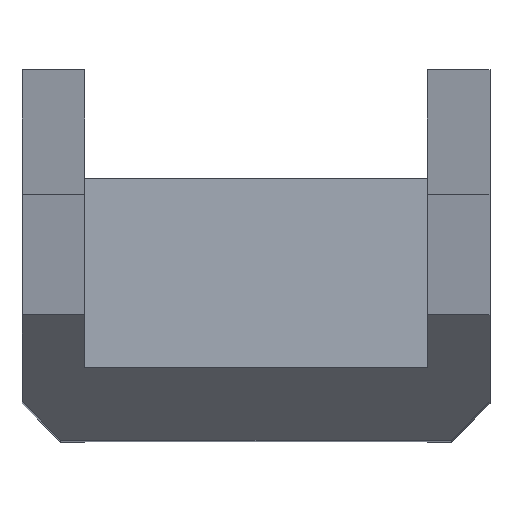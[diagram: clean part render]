
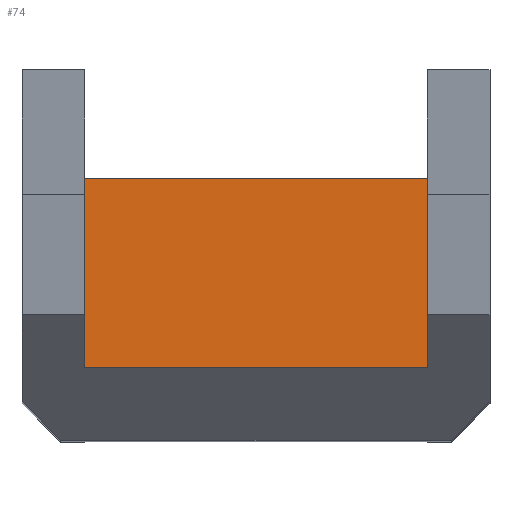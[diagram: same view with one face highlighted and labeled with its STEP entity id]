
A CAD part, top view. The second image highlights one B-rep face of the part: STEP entity #74.
In plain terms, the highlighted planar face has unit normal (0, 0, 1).
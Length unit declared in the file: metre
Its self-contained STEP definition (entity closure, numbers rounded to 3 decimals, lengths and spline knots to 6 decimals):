
#74 = ADVANCED_FACE( '', ( #159 ), #160, .T. );
#159 = FACE_OUTER_BOUND( '', #250, .T. );
#160 = PLANE( '', #251 );
#250 = EDGE_LOOP( '', ( #400, #401, #402, #403 ) );
#251 = AXIS2_PLACEMENT_3D( '', #404, #405, #406 );
#400 = ORIENTED_EDGE( '', *, *, #570, .F. );
#401 = ORIENTED_EDGE( '', *, *, #597, .F. );
#402 = ORIENTED_EDGE( '', *, *, #598, .T. );
#403 = ORIENTED_EDGE( '', *, *, #599, .T. );
#404 = CARTESIAN_POINT( '', ( 0.0089, 0.0099, 0.028708 ) );
#405 = DIRECTION( '', ( 0., 0., 1. ) );
#406 = DIRECTION( '', ( 1., 0., 0. ) );
#570 = EDGE_CURVE( '', #688, #690, #691, .T. );
#597 = EDGE_CURVE( '', #732, #688, #733, .T. );
#598 = EDGE_CURVE( '', #732, #734, #735, .T. );
#599 = EDGE_CURVE( '', #734, #690, #736, .T. );
#688 = VERTEX_POINT( '', #851 );
#690 = VERTEX_POINT( '', #854 );
#691 = LINE( '', #855, #856 );
#732 = VERTEX_POINT( '', #916 );
#733 = LINE( '', #917, #918 );
#734 = VERTEX_POINT( '', #919 );
#735 = LINE( '', #920, #921 );
#736 = LINE( '', #922, #923 );
#851 = CARTESIAN_POINT( '', ( 0.0178, 0., 0.028708 ) );
#854 = CARTESIAN_POINT( '', ( 0., 0., 0.028708 ) );
#855 = CARTESIAN_POINT( '', ( 0.0089, 0., 0.028708 ) );
#856 = VECTOR( '', #1021, 1. );
#916 = CARTESIAN_POINT( '', ( 0.0178, 0.0099, 0.028708 ) );
#917 = CARTESIAN_POINT( '', ( 0.0178, 0.0099, 0.028708 ) );
#918 = VECTOR( '', #1044, 1. );
#919 = CARTESIAN_POINT( '', ( 0., 0.0099, 0.028708 ) );
#920 = CARTESIAN_POINT( '', ( 0.0089, 0.0099, 0.028708 ) );
#921 = VECTOR( '', #1045, 1. );
#922 = CARTESIAN_POINT( '', ( 0., 0.0099, 0.028708 ) );
#923 = VECTOR( '', #1046, 1. );
#1021 = DIRECTION( '', ( -1., 0., 0. ) );
#1044 = DIRECTION( '', ( 0., -1., 0. ) );
#1045 = DIRECTION( '', ( -1., 0., 0. ) );
#1046 = DIRECTION( '', ( 0., -1., 0. ) );
